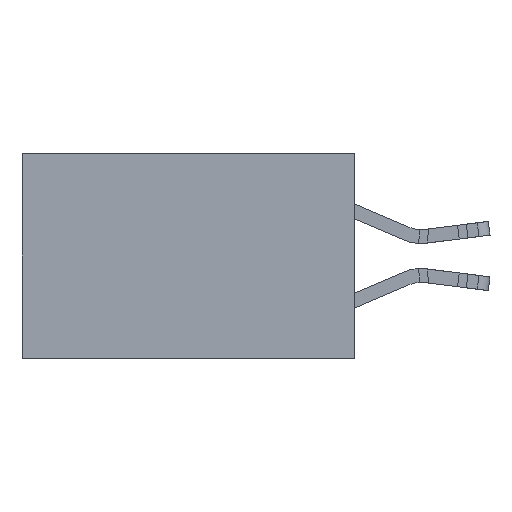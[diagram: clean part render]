
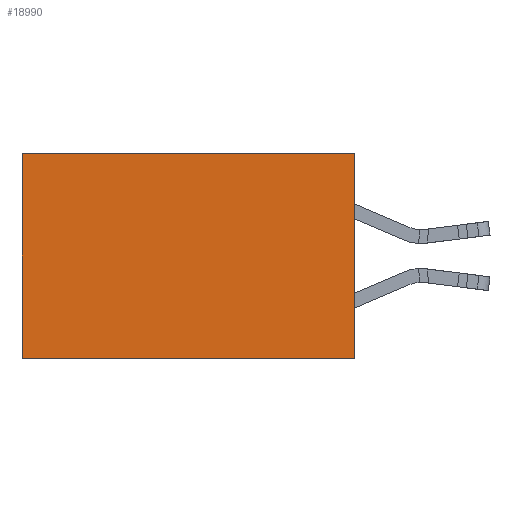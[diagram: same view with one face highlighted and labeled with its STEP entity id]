
A CAD part, left-side view. The second image highlights one B-rep face of the part: STEP entity #18990.
In plain terms, the highlighted planar face has unit normal (-1, 0, 0).
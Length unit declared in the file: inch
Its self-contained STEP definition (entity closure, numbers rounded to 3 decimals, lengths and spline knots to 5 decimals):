
#402 = VERTEX_POINT ( 'NONE', #6250 ) ;
#549 = CARTESIAN_POINT ( 'NONE',  ( 0.298, 0., 0. ) ) ;
#1866 = LINE ( 'NONE', #24114, #27474 ) ;
#3180 = ORIENTED_EDGE ( 'NONE', *, *, #13180, .F. ) ;
#4140 = VERTEX_POINT ( 'NONE', #28903 ) ;
#5519 = ORIENTED_EDGE ( 'NONE', *, *, #23024, .T. ) ;
#6250 = CARTESIAN_POINT ( 'NONE',  ( 0.298, 0., -0.37 ) ) ;
#6667 = DIRECTION ( 'NONE',  ( 0., 1., 0. ) ) ;
#8054 = LINE ( 'NONE', #25327, #13849 ) ;
#8438 = VERTEX_POINT ( 'NONE', #20849 ) ;
#10695 = ORIENTED_EDGE ( 'NONE', *, *, #27059, .F. ) ;
#11396 = DIRECTION ( 'NONE',  ( 1., 0., 0. ) ) ;
#13116 = DIRECTION ( 'NONE',  ( 0., 0., -1. ) ) ;
#13180 = EDGE_CURVE ( 'NONE', #15106, #402, #20216, .T. ) ;
#13656 = VECTOR ( 'NONE', #15637, 39.37008 ) ;
#13849 = VECTOR ( 'NONE', #13116, 39.37008 ) ;
#13897 = EDGE_LOOP ( 'NONE', ( #21178, #10695, #3180, #5519 ) ) ;
#14740 = VECTOR ( 'NONE', #6667, 39.37008 ) ;
#15106 = VERTEX_POINT ( 'NONE', #24957 ) ;
#15637 = DIRECTION ( 'NONE',  ( 0., 0., -1. ) ) ;
#18772 = EDGE_CURVE ( 'NONE', #8438, #4140, #8054, .T. ) ;
#18990 = ADVANCED_FACE ( 'NONE', ( #20801 ), #21202, .F. ) ;
#19034 = CARTESIAN_POINT ( 'NONE',  ( 0.298, 0., 0. ) ) ;
#20216 = LINE ( 'NONE', #549, #13656 ) ;
#20587 = AXIS2_PLACEMENT_3D ( 'NONE', #25935, #11396, #28444 ) ;
#20801 = FACE_OUTER_BOUND ( 'NONE', #13897, .T. ) ;
#20849 = CARTESIAN_POINT ( 'NONE',  ( 0.298, 0.6, 0. ) ) ;
#21178 = ORIENTED_EDGE ( 'NONE', *, *, #18772, .T. ) ;
#21202 = PLANE ( 'NONE',  #20587 ) ;
#23024 = EDGE_CURVE ( 'NONE', #15106, #8438, #29197, .T. ) ;
#24114 = CARTESIAN_POINT ( 'NONE',  ( 0.298, 0., -0.37 ) ) ;
#24957 = CARTESIAN_POINT ( 'NONE',  ( 0.298, 0., 0. ) ) ;
#25327 = CARTESIAN_POINT ( 'NONE',  ( 0.298, 0.6, 0. ) ) ;
#25935 = CARTESIAN_POINT ( 'NONE',  ( 0.298, 0., 0. ) ) ;
#27059 = EDGE_CURVE ( 'NONE', #402, #4140, #1866, .T. ) ;
#27474 = VECTOR ( 'NONE', #31335, 39.37008 ) ;
#28444 = DIRECTION ( 'NONE',  ( 0., 0., -1. ) ) ;
#28903 = CARTESIAN_POINT ( 'NONE',  ( 0.298, 0.6, -0.37 ) ) ;
#29197 = LINE ( 'NONE', #19034, #14740 ) ;
#31335 = DIRECTION ( 'NONE',  ( 0., 1., 0. ) ) ;
